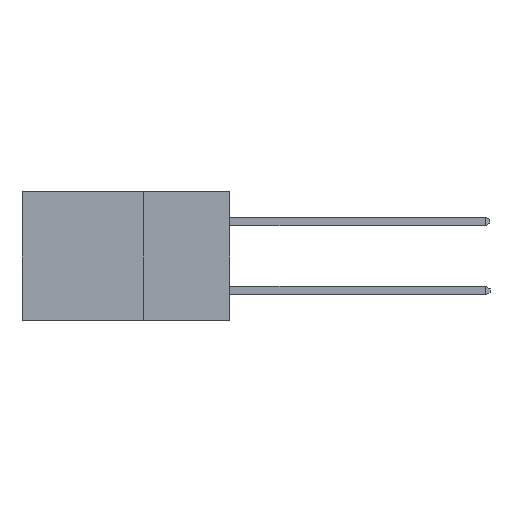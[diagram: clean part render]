
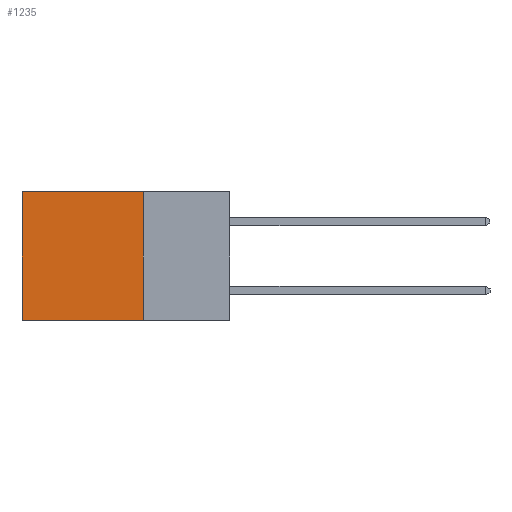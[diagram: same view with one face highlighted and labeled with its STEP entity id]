
A CAD part, left-side view. The second image highlights one B-rep face of the part: STEP entity #1235.
In plain terms, the highlighted planar face has unit normal (-1, 0, 0).
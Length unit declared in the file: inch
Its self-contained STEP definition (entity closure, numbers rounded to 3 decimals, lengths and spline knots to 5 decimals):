
#129 = FACE_OUTER_BOUND ( 'NONE', #2550, .T. ) ;
#393 = ORIENTED_EDGE ( 'NONE', *, *, #6094, .F. ) ;
#910 = VERTEX_POINT ( 'NONE', #3937 ) ;
#991 = DIRECTION ( 'NONE',  ( 0., 0., -1. ) ) ;
#1235 = ADVANCED_FACE ( 'NONE', ( #129 ), #8524, .F. ) ;
#1270 = CARTESIAN_POINT ( 'NONE',  ( 0.2615, 0.6, 0. ) ) ;
#1278 = CARTESIAN_POINT ( 'NONE',  ( 0.2615, 0.25, -0.37 ) ) ;
#1334 = EDGE_CURVE ( 'NONE', #8940, #9739, #2382, .T. ) ;
#1746 = DIRECTION ( 'NONE',  ( 0., 0., -1. ) ) ;
#1888 = VECTOR ( 'NONE', #3662, 39.37008 ) ;
#1959 = DIRECTION ( 'NONE',  ( 0., 0., -1. ) ) ;
#1979 = DIRECTION ( 'NONE',  ( 1., 0., 0. ) ) ;
#2322 = VECTOR ( 'NONE', #1959, 39.37008 ) ;
#2326 = CARTESIAN_POINT ( 'NONE',  ( 0.2615, 0.25, -0.37 ) ) ;
#2382 = LINE ( 'NONE', #6089, #1888 ) ;
#2550 = EDGE_LOOP ( 'NONE', ( #9491, #9735, #393, #6187 ) ) ;
#2723 = CARTESIAN_POINT ( 'NONE',  ( 0.2615, 0.25, 0. ) ) ;
#2913 = LINE ( 'NONE', #8075, #2322 ) ;
#3097 = AXIS2_PLACEMENT_3D ( 'NONE', #1278, #1979, #1746 ) ;
#3099 = DIRECTION ( 'NONE',  ( 0., 1., 0. ) ) ;
#3662 = DIRECTION ( 'NONE',  ( 0., 1., 0. ) ) ;
#3937 = CARTESIAN_POINT ( 'NONE',  ( 0.2615, 0.6, -0.37 ) ) ;
#3986 = LINE ( 'NONE', #2326, #5579 ) ;
#4517 = EDGE_CURVE ( 'NONE', #6425, #910, #3986, .T. ) ;
#5579 = VECTOR ( 'NONE', #3099, 39.37008 ) ;
#6089 = CARTESIAN_POINT ( 'NONE',  ( 0.2615, 0.25, 0. ) ) ;
#6094 = EDGE_CURVE ( 'NONE', #8940, #6425, #7333, .T. ) ;
#6187 = ORIENTED_EDGE ( 'NONE', *, *, #1334, .T. ) ;
#6276 = CARTESIAN_POINT ( 'NONE',  ( 0.2615, 0.25, -0.37 ) ) ;
#6360 = CARTESIAN_POINT ( 'NONE',  ( 0.2615, 0.25, -0.37 ) ) ;
#6375 = VECTOR ( 'NONE', #991, 39.37008 ) ;
#6425 = VERTEX_POINT ( 'NONE', #6276 ) ;
#7333 = LINE ( 'NONE', #6360, #6375 ) ;
#8075 = CARTESIAN_POINT ( 'NONE',  ( 0.2615, 0.6, -0.37 ) ) ;
#8333 = EDGE_CURVE ( 'NONE', #9739, #910, #2913, .T. ) ;
#8524 = PLANE ( 'NONE',  #3097 ) ;
#8940 = VERTEX_POINT ( 'NONE', #2723 ) ;
#9491 = ORIENTED_EDGE ( 'NONE', *, *, #8333, .T. ) ;
#9735 = ORIENTED_EDGE ( 'NONE', *, *, #4517, .F. ) ;
#9739 = VERTEX_POINT ( 'NONE', #1270 ) ;
